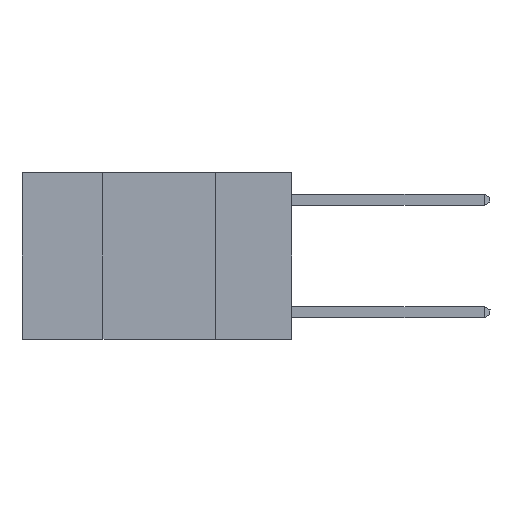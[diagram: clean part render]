
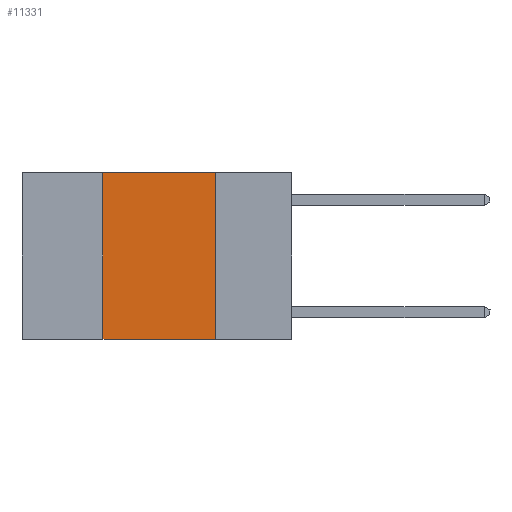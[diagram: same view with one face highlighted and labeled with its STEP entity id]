
A CAD part, left-side view. The second image highlights one B-rep face of the part: STEP entity #11331.
In plain terms, the highlighted planar face has unit normal (-1, 0, 0).
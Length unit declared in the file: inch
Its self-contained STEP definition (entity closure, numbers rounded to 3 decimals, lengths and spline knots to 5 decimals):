
#131 = ORIENTED_EDGE ( 'NONE', *, *, #19276, .F. ) ;
#521 = ORIENTED_EDGE ( 'NONE', *, *, #25829, .F. ) ;
#837 = VECTOR ( 'NONE', #16821, 39.37008 ) ;
#1956 = ORIENTED_EDGE ( 'NONE', *, *, #15507, .F. ) ;
#2131 = VECTOR ( 'NONE', #6133, 39.37008 ) ;
#2240 = CARTESIAN_POINT ( 'NONE',  ( 0., 0.42, 0. ) ) ;
#2364 = ORIENTED_EDGE ( 'NONE', *, *, #24962, .T. ) ;
#4046 = CARTESIAN_POINT ( 'NONE',  ( 0., 0.6, 0. ) ) ;
#5393 = VERTEX_POINT ( 'NONE', #12111 ) ;
#5921 = LINE ( 'NONE', #2240, #837 ) ;
#6133 = DIRECTION ( 'NONE',  ( 0., -1., 0. ) ) ;
#8705 = VERTEX_POINT ( 'NONE', #23072 ) ;
#9101 = DIRECTION ( 'NONE',  ( 1., 0., 0. ) ) ;
#9132 = VECTOR ( 'NONE', #16143, 39.37008 ) ;
#10506 = LINE ( 'NONE', #18766, #23107 ) ;
#11331 = ADVANCED_FACE ( 'NONE', ( #28383 ), #23312, .F. ) ;
#11577 = DIRECTION ( 'NONE',  ( 0., 0., -1. ) ) ;
#12111 = CARTESIAN_POINT ( 'NONE',  ( 0., 0.17, -0.37 ) ) ;
#12694 = EDGE_LOOP ( 'NONE', ( #131, #521, #1956, #2364 ) ) ;
#13693 = VERTEX_POINT ( 'NONE', #19628 ) ;
#15127 = LINE ( 'NONE', #20518, #2131 ) ;
#15507 = EDGE_CURVE ( 'NONE', #17070, #13693, #5921, .T. ) ;
#16143 = DIRECTION ( 'NONE',  ( 0., -1., 0. ) ) ;
#16821 = DIRECTION ( 'NONE',  ( 0., 0., 1. ) ) ;
#17070 = VERTEX_POINT ( 'NONE', #21143 ) ;
#18620 = CARTESIAN_POINT ( 'NONE',  ( 0., 0.6, 0. ) ) ;
#18766 = CARTESIAN_POINT ( 'NONE',  ( 0., 0.17, 0. ) ) ;
#19276 = EDGE_CURVE ( 'NONE', #8705, #5393, #10506, .T. ) ;
#19562 = AXIS2_PLACEMENT_3D ( 'NONE', #18620, #9101, #25642 ) ;
#19628 = CARTESIAN_POINT ( 'NONE',  ( 0., 0.42, 0. ) ) ;
#20518 = CARTESIAN_POINT ( 'NONE',  ( 0., 0.6, -0.37 ) ) ;
#21143 = CARTESIAN_POINT ( 'NONE',  ( 0., 0.42, -0.37 ) ) ;
#21784 = LINE ( 'NONE', #4046, #9132 ) ;
#23072 = CARTESIAN_POINT ( 'NONE',  ( 0., 0.17, 0. ) ) ;
#23107 = VECTOR ( 'NONE', #11577, 39.37008 ) ;
#23312 = PLANE ( 'NONE',  #19562 ) ;
#24962 = EDGE_CURVE ( 'NONE', #17070, #5393, #15127, .T. ) ;
#25642 = DIRECTION ( 'NONE',  ( 0., 0., -1. ) ) ;
#25829 = EDGE_CURVE ( 'NONE', #13693, #8705, #21784, .T. ) ;
#28383 = FACE_OUTER_BOUND ( 'NONE', #12694, .T. ) ;
